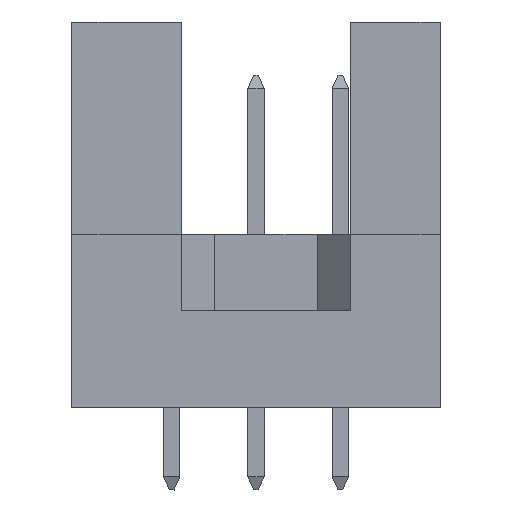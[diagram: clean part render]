
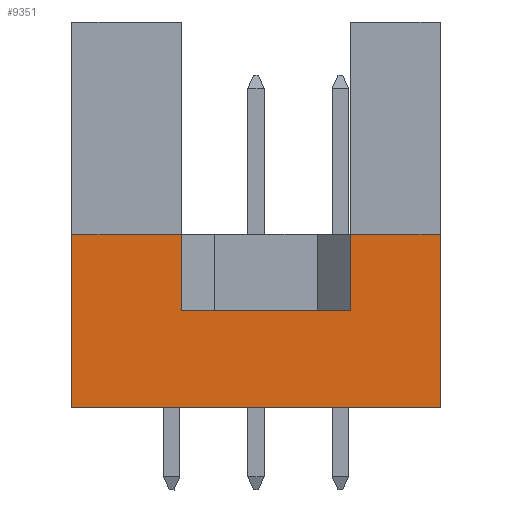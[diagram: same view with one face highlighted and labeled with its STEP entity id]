
A CAD part, left-side view. The second image highlights one B-rep face of the part: STEP entity #9351.
In plain terms, the highlighted planar face has unit normal (-1, 0, 0).
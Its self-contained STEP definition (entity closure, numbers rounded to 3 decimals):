
#24 = VERTEX_POINT ( 'NONE', #3892 ) ;
#106 = ORIENTED_EDGE ( 'NONE', *, *, #154, .F. ) ;
#154 = EDGE_CURVE ( 'NONE', #9973, #24, #8173, .T. ) ;
#164 = LINE ( 'NONE', #999, #2437 ) ;
#311 = CARTESIAN_POINT ( 'NONE',  ( -27.5, 7.79, 5.2 ) ) ;
#715 = CARTESIAN_POINT ( 'NONE',  ( -27.5, 11.1, 0. ) ) ;
#999 = CARTESIAN_POINT ( 'NONE',  ( -27.5, 11.1, 5.2 ) ) ;
#1186 = EDGE_CURVE ( 'NONE', #5570, #3291, #8700, .T. ) ;
#1257 = VERTEX_POINT ( 'NONE', #2448 ) ;
#1592 = VECTOR ( 'NONE', #6704, 1000. ) ;
#1719 = VERTEX_POINT ( 'NONE', #9028 ) ;
#1827 = LINE ( 'NONE', #9855, #3225 ) ;
#2297 = LINE ( 'NONE', #5392, #8825 ) ;
#2437 = VECTOR ( 'NONE', #9237, 1000. ) ;
#2448 = CARTESIAN_POINT ( 'NONE',  ( -27.5, 0., 0. ) ) ;
#2471 = PLANE ( 'NONE',  #6627 ) ;
#2538 = EDGE_CURVE ( 'NONE', #5570, #9973, #2883, .T. ) ;
#2563 = VECTOR ( 'NONE', #6087, 1000. ) ;
#2699 = VERTEX_POINT ( 'NONE', #9667 ) ;
#2883 = LINE ( 'NONE', #6833, #2563 ) ;
#2916 = VERTEX_POINT ( 'NONE', #6716 ) ;
#2977 = CARTESIAN_POINT ( 'NONE',  ( -27.5, 7.79, 2.9 ) ) ;
#3185 = EDGE_CURVE ( 'NONE', #24, #2916, #1827, .T. ) ;
#3225 = VECTOR ( 'NONE', #5185, 1000. ) ;
#3254 = FACE_OUTER_BOUND ( 'NONE', #4989, .T. ) ;
#3291 = VERTEX_POINT ( 'NONE', #311 ) ;
#3333 = CARTESIAN_POINT ( 'NONE',  ( -27.5, 7.79, 2.9 ) ) ;
#3497 = LINE ( 'NONE', #3659, #1592 ) ;
#3659 = CARTESIAN_POINT ( 'NONE',  ( -27.5, 0., 0. ) ) ;
#3892 = CARTESIAN_POINT ( 'NONE',  ( -27.5, 2.71, 5.2 ) ) ;
#4764 = ORIENTED_EDGE ( 'NONE', *, *, #6824, .F. ) ;
#4843 = CARTESIAN_POINT ( 'NONE',  ( -27.5, 2.71, 2.9 ) ) ;
#4881 = DIRECTION ( 'NONE',  ( 1., 0., 0. ) ) ;
#4989 = EDGE_LOOP ( 'NONE', ( #6547, #7861, #8877, #4764, #10061, #5685, #9723, #106 ) ) ;
#5131 = VECTOR ( 'NONE', #6970, 1000. ) ;
#5185 = DIRECTION ( 'NONE',  ( 0., -1., 0. ) ) ;
#5392 = CARTESIAN_POINT ( 'NONE',  ( -27.5, 11.1, 0. ) ) ;
#5570 = VERTEX_POINT ( 'NONE', #3333 ) ;
#5673 = CARTESIAN_POINT ( 'NONE',  ( -27.5, 11.1, 0. ) ) ;
#5685 = ORIENTED_EDGE ( 'NONE', *, *, #8465, .T. ) ;
#6087 = DIRECTION ( 'NONE',  ( 0., -1., 0. ) ) ;
#6525 = EDGE_CURVE ( 'NONE', #2699, #3291, #164, .T. ) ;
#6547 = ORIENTED_EDGE ( 'NONE', *, *, #2538, .F. ) ;
#6627 = AXIS2_PLACEMENT_3D ( 'NONE', #5673, #4881, #8097 ) ;
#6704 = DIRECTION ( 'NONE',  ( 0., 0., 1. ) ) ;
#6716 = CARTESIAN_POINT ( 'NONE',  ( -27.5, 0., 5.2 ) ) ;
#6824 = EDGE_CURVE ( 'NONE', #1719, #2699, #2297, .T. ) ;
#6833 = CARTESIAN_POINT ( 'NONE',  ( -27.5, 7.79, 2.9 ) ) ;
#6955 = VECTOR ( 'NONE', #9427, 1000. ) ;
#6970 = DIRECTION ( 'NONE',  ( 0., 0., 1. ) ) ;
#7416 = CARTESIAN_POINT ( 'NONE',  ( -27.5, 2.71, 2.9 ) ) ;
#7861 = ORIENTED_EDGE ( 'NONE', *, *, #1186, .T. ) ;
#8097 = DIRECTION ( 'NONE',  ( 0., 0., -1. ) ) ;
#8173 = LINE ( 'NONE', #4843, #10091 ) ;
#8465 = EDGE_CURVE ( 'NONE', #1257, #2916, #3497, .T. ) ;
#8577 = EDGE_CURVE ( 'NONE', #1719, #1257, #8698, .T. ) ;
#8608 = DIRECTION ( 'NONE',  ( 0., 0., 1. ) ) ;
#8698 = LINE ( 'NONE', #715, #6955 ) ;
#8700 = LINE ( 'NONE', #2977, #5131 ) ;
#8825 = VECTOR ( 'NONE', #8608, 1000. ) ;
#8877 = ORIENTED_EDGE ( 'NONE', *, *, #6525, .F. ) ;
#9003 = DIRECTION ( 'NONE',  ( 0., 0., 1. ) ) ;
#9028 = CARTESIAN_POINT ( 'NONE',  ( -27.5, 11.1, 0. ) ) ;
#9237 = DIRECTION ( 'NONE',  ( 0., -1., 0. ) ) ;
#9351 = ADVANCED_FACE ( 'NONE', ( #3254 ), #2471, .F. ) ;
#9427 = DIRECTION ( 'NONE',  ( 0., -1., 0. ) ) ;
#9667 = CARTESIAN_POINT ( 'NONE',  ( -27.5, 11.1, 5.2 ) ) ;
#9723 = ORIENTED_EDGE ( 'NONE', *, *, #3185, .F. ) ;
#9855 = CARTESIAN_POINT ( 'NONE',  ( -27.5, 11.1, 5.2 ) ) ;
#9973 = VERTEX_POINT ( 'NONE', #7416 ) ;
#10061 = ORIENTED_EDGE ( 'NONE', *, *, #8577, .T. ) ;
#10091 = VECTOR ( 'NONE', #9003, 1000. ) ;
